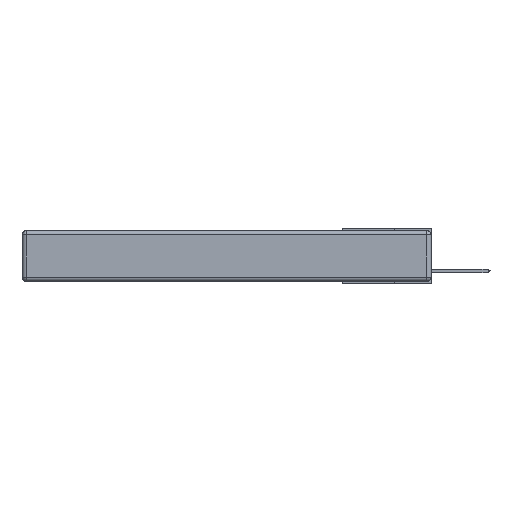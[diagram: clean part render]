
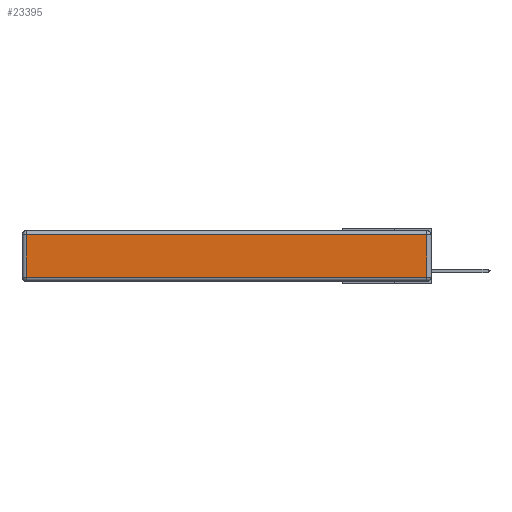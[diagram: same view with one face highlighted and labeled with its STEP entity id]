
A CAD part, left-side view. The second image highlights one B-rep face of the part: STEP entity #23395.
In plain terms, the highlighted planar face has unit normal (-1, 0, 0).
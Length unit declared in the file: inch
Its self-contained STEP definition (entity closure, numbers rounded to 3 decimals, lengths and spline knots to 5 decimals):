
#42 = DIRECTION ( 'NONE',  ( 0., -1., 0. ) ) ;
#1586 = EDGE_CURVE ( 'NONE', #28760, #14150, #22159, .T. ) ;
#2535 = DIRECTION ( 'NONE',  ( 0., 0., 1. ) ) ;
#3084 = VECTOR ( 'NONE', #2535, 39.37008 ) ;
#5036 = DIRECTION ( 'NONE',  ( -1., 0., 0. ) ) ;
#6403 = EDGE_CURVE ( 'NONE', #11126, #28760, #12306, .T. ) ;
#6510 = VECTOR ( 'NONE', #18838, 39.37008 ) ;
#8230 = ORIENTED_EDGE ( 'NONE', *, *, #10333, .T. ) ;
#8285 = ORIENTED_EDGE ( 'NONE', *, *, #6403, .T. ) ;
#9717 = CARTESIAN_POINT ( 'NONE',  ( 0., 0., -0.343 ) ) ;
#9889 = CARTESIAN_POINT ( 'NONE',  ( 0., 2.72, -0.03 ) ) ;
#10333 = EDGE_CURVE ( 'NONE', #14150, #10614, #22997, .T. ) ;
#10614 = VERTEX_POINT ( 'NONE', #9889 ) ;
#11126 = VERTEX_POINT ( 'NONE', #27348 ) ;
#11499 = AXIS2_PLACEMENT_3D ( 'NONE', #9717, #5036, #30939 ) ;
#11782 = CARTESIAN_POINT ( 'NONE',  ( 0., 2.75, -0.03 ) ) ;
#12171 = DIRECTION ( 'NONE',  ( 0., 0., -1. ) ) ;
#12306 = LINE ( 'NONE', #14322, #28389 ) ;
#12425 = CARTESIAN_POINT ( 'NONE',  ( 0., 0.03, -0.313 ) ) ;
#12773 = ORIENTED_EDGE ( 'NONE', *, *, #29430, .T. ) ;
#14150 = VERTEX_POINT ( 'NONE', #18960 ) ;
#14322 = CARTESIAN_POINT ( 'NONE',  ( 0., 0., -0.313 ) ) ;
#14426 = PLANE ( 'NONE',  #11499 ) ;
#14672 = CARTESIAN_POINT ( 'NONE',  ( 0., 2.72, -0.343 ) ) ;
#17445 = VECTOR ( 'NONE', #12171, 39.37008 ) ;
#18838 = DIRECTION ( 'NONE',  ( 0., 1., 0. ) ) ;
#18960 = CARTESIAN_POINT ( 'NONE',  ( 0., 0.03, -0.03 ) ) ;
#21504 = EDGE_LOOP ( 'NONE', ( #8285, #27685, #8230, #12773 ) ) ;
#22159 = LINE ( 'NONE', #24176, #3084 ) ;
#22997 = LINE ( 'NONE', #11782, #6510 ) ;
#23395 = ADVANCED_FACE ( 'NONE', ( #24672 ), #14426, .T. ) ;
#24176 = CARTESIAN_POINT ( 'NONE',  ( 0., 0.03, -0.343 ) ) ;
#24672 = FACE_OUTER_BOUND ( 'NONE', #21504, .T. ) ;
#27348 = CARTESIAN_POINT ( 'NONE',  ( 0., 2.72, -0.313 ) ) ;
#27685 = ORIENTED_EDGE ( 'NONE', *, *, #1586, .T. ) ;
#28389 = VECTOR ( 'NONE', #42, 39.37008 ) ;
#28760 = VERTEX_POINT ( 'NONE', #12425 ) ;
#29430 = EDGE_CURVE ( 'NONE', #10614, #11126, #30119, .T. ) ;
#30119 = LINE ( 'NONE', #14672, #17445 ) ;
#30939 = DIRECTION ( 'NONE',  ( 0., 0., 1. ) ) ;
